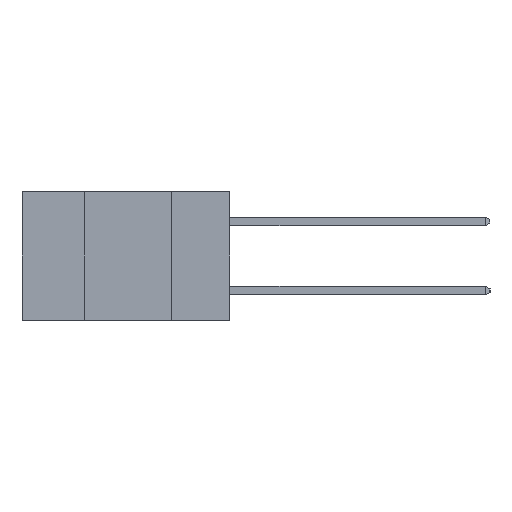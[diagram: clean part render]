
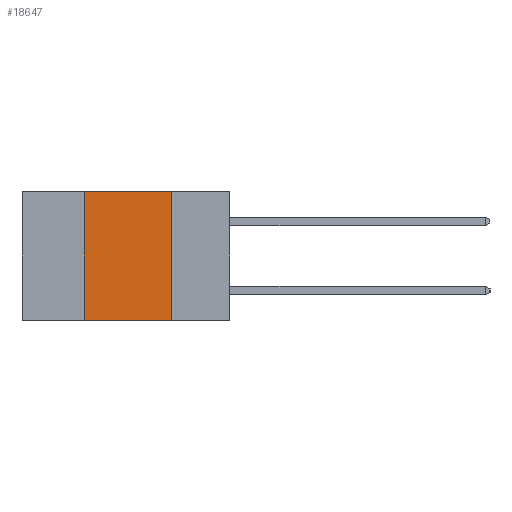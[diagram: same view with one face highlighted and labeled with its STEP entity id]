
A CAD part, left-side view. The second image highlights one B-rep face of the part: STEP entity #18647.
In plain terms, the highlighted planar face has unit normal (-1, 0, 0).
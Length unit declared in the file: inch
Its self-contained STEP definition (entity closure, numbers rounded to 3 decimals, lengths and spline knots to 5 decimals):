
#517 = DIRECTION ( 'NONE',  ( 0., -1., 0. ) ) ;
#656 = ORIENTED_EDGE ( 'NONE', *, *, #5332, .F. ) ;
#843 = CARTESIAN_POINT ( 'NONE',  ( 0., 0.42, 0. ) ) ;
#913 = EDGE_CURVE ( 'NONE', #9600, #15516, #16589, .T. ) ;
#2326 = CARTESIAN_POINT ( 'NONE',  ( 0., 0.17, 0. ) ) ;
#3729 = CARTESIAN_POINT ( 'NONE',  ( 0., 0.17, -0.37 ) ) ;
#4068 = DIRECTION ( 'NONE',  ( 0., 0., -1. ) ) ;
#4251 = VECTOR ( 'NONE', #517, 39.37008 ) ;
#4289 = CARTESIAN_POINT ( 'NONE',  ( 0., 0.17, -0.37 ) ) ;
#4320 = VECTOR ( 'NONE', #4476, 39.37008 ) ;
#4476 = DIRECTION ( 'NONE',  ( 0., 0., 1. ) ) ;
#4894 = CARTESIAN_POINT ( 'NONE',  ( 0., 0.42, -0.37 ) ) ;
#5023 = ORIENTED_EDGE ( 'NONE', *, *, #913, .T. ) ;
#5295 = EDGE_CURVE ( 'NONE', #9600, #15454, #18849, .T. ) ;
#5332 = EDGE_CURVE ( 'NONE', #17105, #15516, #8559, .T. ) ;
#6233 = PLANE ( 'NONE',  #15362 ) ;
#7509 = LINE ( 'NONE', #7955, #11315 ) ;
#7779 = CARTESIAN_POINT ( 'NONE',  ( 0., 0.6, 0. ) ) ;
#7846 = DIRECTION ( 'NONE',  ( 0., 0., -1. ) ) ;
#7955 = CARTESIAN_POINT ( 'NONE',  ( 0., 0.6, 0. ) ) ;
#8023 = ORIENTED_EDGE ( 'NONE', *, *, #5295, .F. ) ;
#8559 = LINE ( 'NONE', #3729, #16653 ) ;
#9188 = EDGE_LOOP ( 'NONE', ( #656, #12308, #8023, #5023 ) ) ;
#9565 = DIRECTION ( 'NONE',  ( 0., -1., 0. ) ) ;
#9600 = VERTEX_POINT ( 'NONE', #12310 ) ;
#10975 = CARTESIAN_POINT ( 'NONE',  ( 0., 0.6, -0.37 ) ) ;
#11129 = EDGE_CURVE ( 'NONE', #15454, #17105, #7509, .T. ) ;
#11315 = VECTOR ( 'NONE', #9565, 39.37008 ) ;
#12308 = ORIENTED_EDGE ( 'NONE', *, *, #11129, .F. ) ;
#12310 = CARTESIAN_POINT ( 'NONE',  ( 0., 0.42, -0.37 ) ) ;
#12892 = FACE_OUTER_BOUND ( 'NONE', #9188, .T. ) ;
#15362 = AXIS2_PLACEMENT_3D ( 'NONE', #7779, #17497, #7846 ) ;
#15454 = VERTEX_POINT ( 'NONE', #843 ) ;
#15516 = VERTEX_POINT ( 'NONE', #4289 ) ;
#16589 = LINE ( 'NONE', #10975, #4251 ) ;
#16653 = VECTOR ( 'NONE', #4068, 39.37008 ) ;
#17105 = VERTEX_POINT ( 'NONE', #2326 ) ;
#17497 = DIRECTION ( 'NONE',  ( 1., 0., 0. ) ) ;
#18647 = ADVANCED_FACE ( 'NONE', ( #12892 ), #6233, .F. ) ;
#18849 = LINE ( 'NONE', #4894, #4320 ) ;
